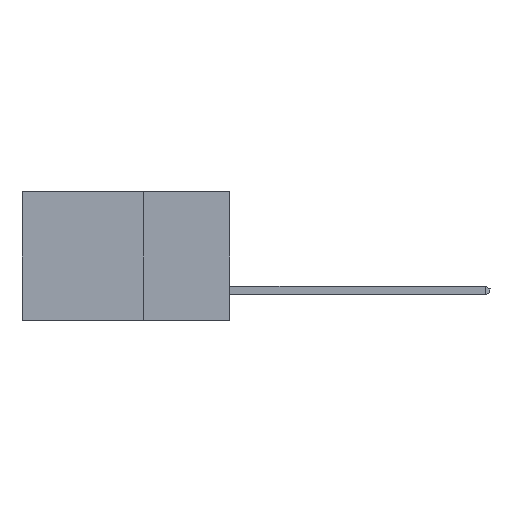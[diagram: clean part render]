
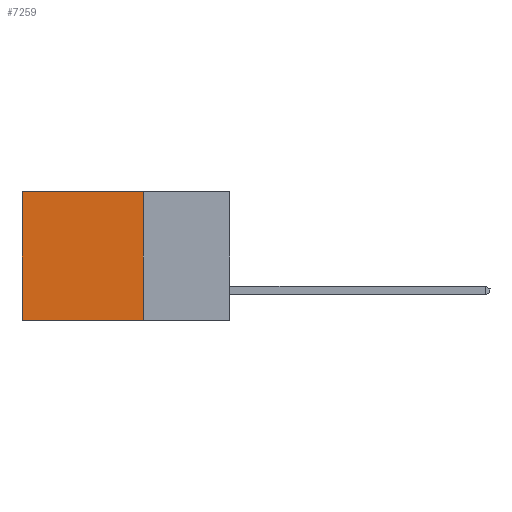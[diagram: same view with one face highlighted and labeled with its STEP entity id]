
A CAD part, left-side view. The second image highlights one B-rep face of the part: STEP entity #7259.
In plain terms, the highlighted planar face has unit normal (-1, 0, 0).
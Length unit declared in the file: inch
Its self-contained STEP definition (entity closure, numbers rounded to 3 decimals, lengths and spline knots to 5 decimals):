
#392 = CARTESIAN_POINT ( 'NONE',  ( 0.2615, 0.25, 0. ) ) ;
#534 = CARTESIAN_POINT ( 'NONE',  ( 0.2615, 0.25, -0.37 ) ) ;
#963 = CARTESIAN_POINT ( 'NONE',  ( 0.2615, 0.25, 0. ) ) ;
#1018 = VERTEX_POINT ( 'NONE', #963 ) ;
#1373 = CARTESIAN_POINT ( 'NONE',  ( 0.2615, 0.6, 0. ) ) ;
#1596 = EDGE_LOOP ( 'NONE', ( #8338, #3777, #2996, #2394 ) ) ;
#2187 = DIRECTION ( 'NONE',  ( 0., 0., -1. ) ) ;
#2354 = LINE ( 'NONE', #534, #4415 ) ;
#2358 = VECTOR ( 'NONE', #2187, 39.37008 ) ;
#2394 = ORIENTED_EDGE ( 'NONE', *, *, #5772, .T. ) ;
#2709 = VECTOR ( 'NONE', #3625, 39.37008 ) ;
#2996 = ORIENTED_EDGE ( 'NONE', *, *, #5293, .F. ) ;
#3398 = LINE ( 'NONE', #7577, #9046 ) ;
#3625 = DIRECTION ( 'NONE',  ( 0., 1., 0. ) ) ;
#3663 = LINE ( 'NONE', #3717, #2358 ) ;
#3717 = CARTESIAN_POINT ( 'NONE',  ( 0.2615, 0.25, -0.37 ) ) ;
#3777 = ORIENTED_EDGE ( 'NONE', *, *, #10668, .F. ) ;
#4415 = VECTOR ( 'NONE', #10742, 39.37008 ) ;
#4554 = PLANE ( 'NONE',  #7592 ) ;
#5293 = EDGE_CURVE ( 'NONE', #1018, #5692, #3663, .T. ) ;
#5373 = VERTEX_POINT ( 'NONE', #1373 ) ;
#5692 = VERTEX_POINT ( 'NONE', #10068 ) ;
#5772 = EDGE_CURVE ( 'NONE', #1018, #5373, #7863, .T. ) ;
#6132 = DIRECTION ( 'NONE',  ( 0., 0., -1. ) ) ;
#7259 = ADVANCED_FACE ( 'NONE', ( #8700 ), #4554, .F. ) ;
#7423 = DIRECTION ( 'NONE',  ( 0., 0., -1. ) ) ;
#7577 = CARTESIAN_POINT ( 'NONE',  ( 0.2615, 0.6, -0.37 ) ) ;
#7592 = AXIS2_PLACEMENT_3D ( 'NONE', #10263, #7864, #6132 ) ;
#7863 = LINE ( 'NONE', #392, #2709 ) ;
#7864 = DIRECTION ( 'NONE',  ( 1., 0., 0. ) ) ;
#7973 = VERTEX_POINT ( 'NONE', #9534 ) ;
#8338 = ORIENTED_EDGE ( 'NONE', *, *, #9042, .T. ) ;
#8700 = FACE_OUTER_BOUND ( 'NONE', #1596, .T. ) ;
#9042 = EDGE_CURVE ( 'NONE', #5373, #7973, #3398, .T. ) ;
#9046 = VECTOR ( 'NONE', #7423, 39.37008 ) ;
#9534 = CARTESIAN_POINT ( 'NONE',  ( 0.2615, 0.6, -0.37 ) ) ;
#10068 = CARTESIAN_POINT ( 'NONE',  ( 0.2615, 0.25, -0.37 ) ) ;
#10263 = CARTESIAN_POINT ( 'NONE',  ( 0.2615, 0.25, -0.37 ) ) ;
#10668 = EDGE_CURVE ( 'NONE', #5692, #7973, #2354, .T. ) ;
#10742 = DIRECTION ( 'NONE',  ( 0., 1., 0. ) ) ;
